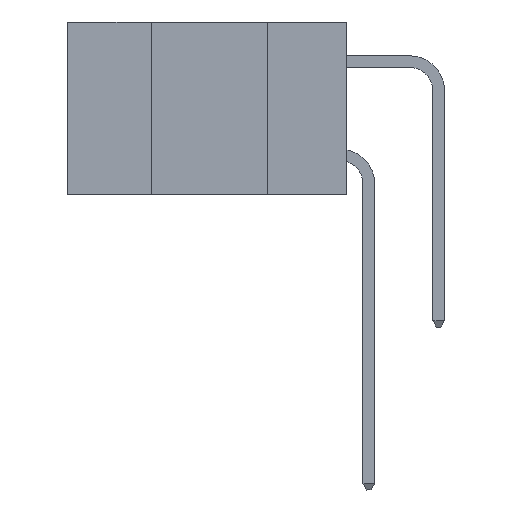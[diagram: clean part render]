
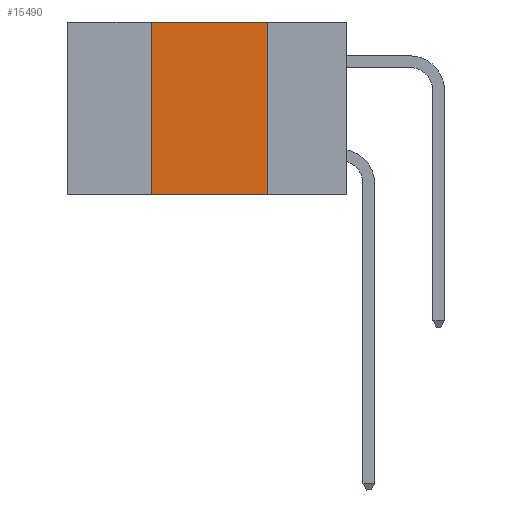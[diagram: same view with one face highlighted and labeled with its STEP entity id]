
A CAD part, left-side view. The second image highlights one B-rep face of the part: STEP entity #15490.
In plain terms, the highlighted planar face has unit normal (-1, 0, 0).
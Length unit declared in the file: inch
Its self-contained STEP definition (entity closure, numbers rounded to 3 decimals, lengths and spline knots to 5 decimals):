
#1498 = CARTESIAN_POINT ( 'NONE',  ( 0., 0.42, 0. ) ) ;
#2056 = LINE ( 'NONE', #19887, #15346 ) ;
#2777 = ORIENTED_EDGE ( 'NONE', *, *, #21310, .T. ) ;
#2785 = DIRECTION ( 'NONE',  ( 0., 0., -1. ) ) ;
#3458 = EDGE_CURVE ( 'NONE', #10653, #18435, #4447, .T. ) ;
#4447 = LINE ( 'NONE', #1498, #21174 ) ;
#6084 = EDGE_CURVE ( 'NONE', #18435, #19928, #16520, .T. ) ;
#7692 = CARTESIAN_POINT ( 'NONE',  ( 0., 0.42, 0. ) ) ;
#8851 = ORIENTED_EDGE ( 'NONE', *, *, #6084, .F. ) ;
#9022 = DIRECTION ( 'NONE',  ( 0., -1., 0. ) ) ;
#10653 = VERTEX_POINT ( 'NONE', #18503 ) ;
#11692 = FACE_OUTER_BOUND ( 'NONE', #18400, .T. ) ;
#11917 = VECTOR ( 'NONE', #9022, 39.37008 ) ;
#12288 = LINE ( 'NONE', #12387, #15269 ) ;
#12387 = CARTESIAN_POINT ( 'NONE',  ( 0., 0.17, 0. ) ) ;
#13051 = DIRECTION ( 'NONE',  ( 0., -1., 0. ) ) ;
#13173 = DIRECTION ( 'NONE',  ( 1., 0., 0. ) ) ;
#14083 = VERTEX_POINT ( 'NONE', #19594 ) ;
#14375 = ORIENTED_EDGE ( 'NONE', *, *, #14668, .F. ) ;
#14668 = EDGE_CURVE ( 'NONE', #19928, #14083, #12288, .T. ) ;
#15269 = VECTOR ( 'NONE', #20923, 39.37008 ) ;
#15346 = VECTOR ( 'NONE', #13051, 39.37008 ) ;
#15490 = ADVANCED_FACE ( 'NONE', ( #11692 ), #18291, .F. ) ;
#16520 = LINE ( 'NONE', #21045, #11917 ) ;
#17081 = DIRECTION ( 'NONE',  ( 0., 0., 1. ) ) ;
#18291 = PLANE ( 'NONE',  #18525 ) ;
#18400 = EDGE_LOOP ( 'NONE', ( #14375, #8851, #18647, #2777 ) ) ;
#18435 = VERTEX_POINT ( 'NONE', #7692 ) ;
#18503 = CARTESIAN_POINT ( 'NONE',  ( 0., 0.42, -0.37 ) ) ;
#18525 = AXIS2_PLACEMENT_3D ( 'NONE', #21686, #13173, #2785 ) ;
#18647 = ORIENTED_EDGE ( 'NONE', *, *, #3458, .F. ) ;
#19594 = CARTESIAN_POINT ( 'NONE',  ( 0., 0.17, -0.37 ) ) ;
#19887 = CARTESIAN_POINT ( 'NONE',  ( 0., 0.6, -0.37 ) ) ;
#19928 = VERTEX_POINT ( 'NONE', #21287 ) ;
#20923 = DIRECTION ( 'NONE',  ( 0., 0., -1. ) ) ;
#21045 = CARTESIAN_POINT ( 'NONE',  ( 0., 0.6, 0. ) ) ;
#21174 = VECTOR ( 'NONE', #17081, 39.37008 ) ;
#21287 = CARTESIAN_POINT ( 'NONE',  ( 0., 0.17, 0. ) ) ;
#21310 = EDGE_CURVE ( 'NONE', #10653, #14083, #2056, .T. ) ;
#21686 = CARTESIAN_POINT ( 'NONE',  ( 0., 0.6, 0. ) ) ;
